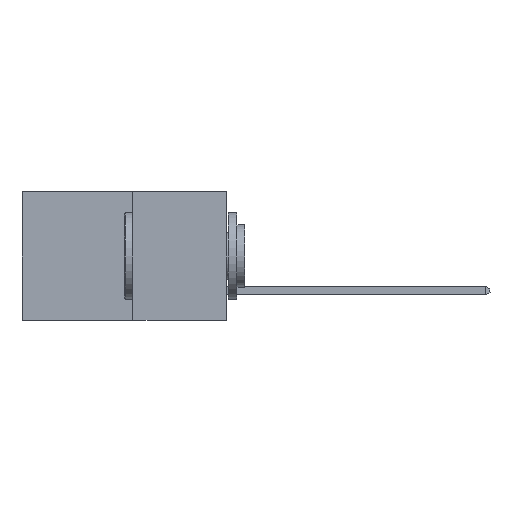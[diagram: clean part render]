
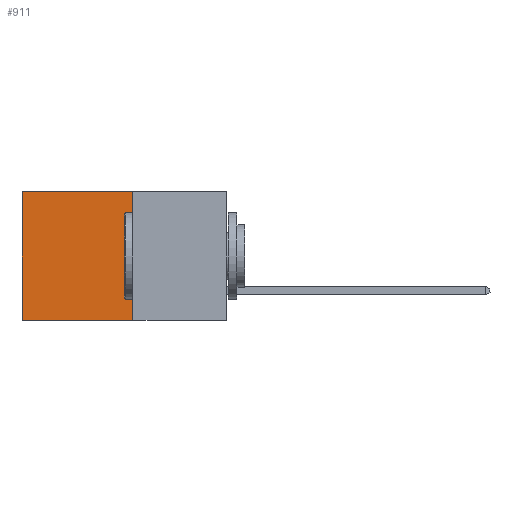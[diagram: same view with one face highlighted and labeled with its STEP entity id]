
A CAD part, left-side view. The second image highlights one B-rep face of the part: STEP entity #911.
In plain terms, the highlighted planar face has unit normal (-1, 0, 0).
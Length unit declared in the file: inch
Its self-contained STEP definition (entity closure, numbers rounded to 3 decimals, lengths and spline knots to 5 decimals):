
#844 = ORIENTED_EDGE ( 'NONE', *, *, #5310, .T. ) ;
#895 = CARTESIAN_POINT ( 'NONE',  ( 0.277, 0.59, -0.37 ) ) ;
#911 = ADVANCED_FACE ( 'NONE', ( #10993 ), #8072, .F. ) ;
#1173 = DIRECTION ( 'NONE',  ( 0., 0., -1. ) ) ;
#1578 = CARTESIAN_POINT ( 'NONE',  ( 0.277, 0.59, -0.37 ) ) ;
#1629 = VERTEX_POINT ( 'NONE', #1578 ) ;
#1639 = EDGE_CURVE ( 'NONE', #8583, #1629, #4118, .T. ) ;
#2104 = CARTESIAN_POINT ( 'NONE',  ( 0.277, 0.27, -0.37 ) ) ;
#2141 = AXIS2_PLACEMENT_3D ( 'NONE', #10497, #3828, #8303 ) ;
#2664 = LINE ( 'NONE', #7066, #7453 ) ;
#3719 = CARTESIAN_POINT ( 'NONE',  ( 0.277, 0.59, 0. ) ) ;
#3828 = DIRECTION ( 'NONE',  ( 1., 0., 0. ) ) ;
#4118 = LINE ( 'NONE', #895, #6727 ) ;
#4339 = EDGE_CURVE ( 'NONE', #7437, #6717, #9686, .T. ) ;
#4631 = ORIENTED_EDGE ( 'NONE', *, *, #6491, .F. ) ;
#4670 = CARTESIAN_POINT ( 'NONE',  ( 0.277, 0.27, -0.37 ) ) ;
#5310 = EDGE_CURVE ( 'NONE', #7437, #8583, #2664, .T. ) ;
#6433 = ORIENTED_EDGE ( 'NONE', *, *, #1639, .T. ) ;
#6491 = EDGE_CURVE ( 'NONE', #6717, #1629, #11237, .T. ) ;
#6586 = VECTOR ( 'NONE', #7027, 39.37008 ) ;
#6717 = VERTEX_POINT ( 'NONE', #4670 ) ;
#6727 = VECTOR ( 'NONE', #8085, 39.37008 ) ;
#6968 = CARTESIAN_POINT ( 'NONE',  ( 0.277, 0.27, -0.37 ) ) ;
#7027 = DIRECTION ( 'NONE',  ( 0., 1., 0. ) ) ;
#7066 = CARTESIAN_POINT ( 'NONE',  ( 0.277, 0.27, 0. ) ) ;
#7157 = DIRECTION ( 'NONE',  ( 0., 1., 0. ) ) ;
#7437 = VERTEX_POINT ( 'NONE', #10778 ) ;
#7453 = VECTOR ( 'NONE', #7157, 39.37008 ) ;
#7819 = ORIENTED_EDGE ( 'NONE', *, *, #4339, .F. ) ;
#8072 = PLANE ( 'NONE',  #2141 ) ;
#8085 = DIRECTION ( 'NONE',  ( 0., 0., -1. ) ) ;
#8303 = DIRECTION ( 'NONE',  ( 0., 0., -1. ) ) ;
#8583 = VERTEX_POINT ( 'NONE', #3719 ) ;
#8939 = EDGE_LOOP ( 'NONE', ( #6433, #4631, #7819, #844 ) ) ;
#9421 = VECTOR ( 'NONE', #1173, 39.37008 ) ;
#9686 = LINE ( 'NONE', #2104, #9421 ) ;
#10497 = CARTESIAN_POINT ( 'NONE',  ( 0.277, 0.27, -0.37 ) ) ;
#10778 = CARTESIAN_POINT ( 'NONE',  ( 0.277, 0.27, 0. ) ) ;
#10993 = FACE_OUTER_BOUND ( 'NONE', #8939, .T. ) ;
#11237 = LINE ( 'NONE', #6968, #6586 ) ;
